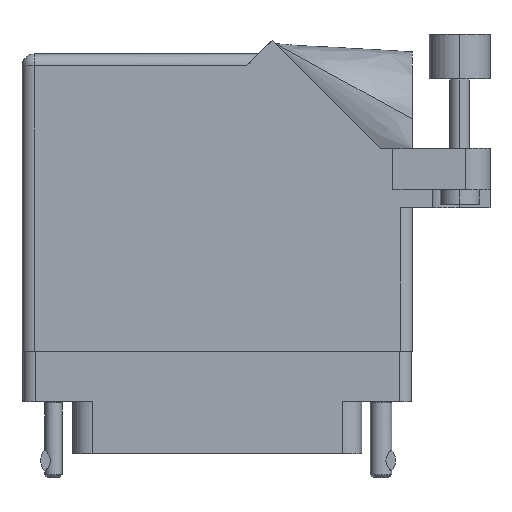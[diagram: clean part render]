
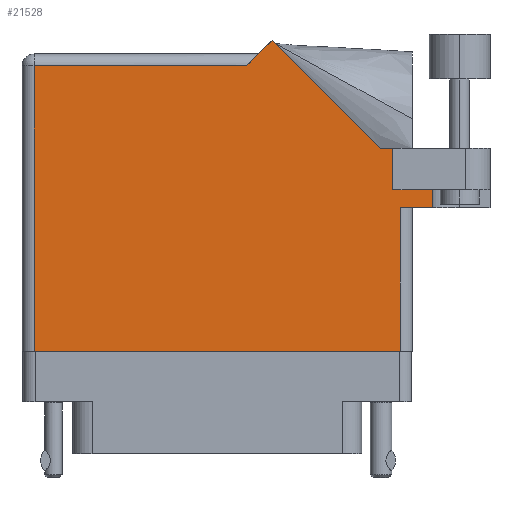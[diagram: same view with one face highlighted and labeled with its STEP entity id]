
A CAD part, front view. The second image highlights one B-rep face of the part: STEP entity #21528.
In plain terms, the highlighted face is planar.
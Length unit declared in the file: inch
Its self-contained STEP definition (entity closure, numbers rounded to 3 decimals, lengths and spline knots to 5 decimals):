
#61 = ORIENTED_EDGE ( 'NONE', *, *, #33246, .T. ) ;
#409 = ORIENTED_EDGE ( 'NONE', *, *, #46826, .F. ) ;
#610 = VERTEX_POINT ( 'NONE', #6853 ) ;
#816 = VERTEX_POINT ( 'NONE', #29741 ) ;
#1516 = DIRECTION ( 'NONE',  ( 0., 1., 0. ) ) ;
#3963 = CARTESIAN_POINT ( 'NONE',  ( 1.84442, 1.044, 0. ) ) ;
#4258 = VERTEX_POINT ( 'NONE', #4443 ) ;
#4443 = CARTESIAN_POINT ( 'NONE',  ( 0.062, 0., 0. ) ) ;
#5103 = DIRECTION ( 'NONE',  ( -0.707, 0.707, 0. ) ) ;
#5452 = ORIENTED_EDGE ( 'NONE', *, *, #24440, .T. ) ;
#6718 = CARTESIAN_POINT ( 'NONE',  ( 1.91, 0.831, 0. ) ) ;
#6816 = CARTESIAN_POINT ( 'NONE',  ( 1.91, 1.044, 0. ) ) ;
#6853 = CARTESIAN_POINT ( 'NONE',  ( 2.1115, 0.831, 0. ) ) ;
#7058 = VERTEX_POINT ( 'NONE', #6816 ) ;
#7632 = CARTESIAN_POINT ( 'NONE',  ( 0., 0., 0. ) ) ;
#8028 = ORIENTED_EDGE ( 'NONE', *, *, #10808, .T. ) ;
#9921 = DIRECTION ( 'NONE',  ( 0., -1., 0. ) ) ;
#10327 = VERTEX_POINT ( 'NONE', #3963 ) ;
#10651 = VECTOR ( 'NONE', #18929, 39.37008 ) ;
#10808 = EDGE_CURVE ( 'NONE', #44671, #12719, #25239, .T. ) ;
#11170 = CARTESIAN_POINT ( 'NONE',  ( 2.1115, 0.737, 0. ) ) ;
#11252 = PLANE ( 'NONE',  #29111 ) ;
#12719 = VERTEX_POINT ( 'NONE', #14755 ) ;
#13970 = CARTESIAN_POINT ( 'NONE',  ( 1.28771, 1.60071, 0. ) ) ;
#14287 = ORIENTED_EDGE ( 'NONE', *, *, #27732, .T. ) ;
#14678 = DIRECTION ( 'NONE',  ( 0., 0., -1. ) ) ;
#14755 = CARTESIAN_POINT ( 'NONE',  ( 1.948, 0.737, 0. ) ) ;
#16064 = DIRECTION ( 'NONE',  ( 1., 0., 0. ) ) ;
#16379 = DIRECTION ( 'NONE',  ( -0.707, -0.707, 0. ) ) ;
#16414 = LINE ( 'NONE', #7632, #10651 ) ;
#18099 = LINE ( 'NONE', #39887, #40368 ) ;
#18368 = CARTESIAN_POINT ( 'NONE',  ( 1.948, 0.737, 0. ) ) ;
#18465 = VERTEX_POINT ( 'NONE', #43264 ) ;
#18929 = DIRECTION ( 'NONE',  ( 1., 0., 0. ) ) ;
#19788 = ORIENTED_EDGE ( 'NONE', *, *, #43448, .T. ) ;
#19998 = CARTESIAN_POINT ( 'NONE',  ( 1.91, 0.831, 0. ) ) ;
#20545 = VECTOR ( 'NONE', #27353, 39.37008 ) ;
#20942 = VECTOR ( 'NONE', #5103, 39.37008 ) ;
#21034 = CARTESIAN_POINT ( 'NONE',  ( 1.948, 0., 0. ) ) ;
#21461 = VECTOR ( 'NONE', #16379, 39.37008 ) ;
#21528 = ADVANCED_FACE ( 'NONE', ( #33737 ), #11252, .F. ) ;
#21626 = DIRECTION ( 'NONE',  ( -1., 0., 0. ) ) ;
#21984 = LINE ( 'NONE', #31185, #29567 ) ;
#22434 = VECTOR ( 'NONE', #1516, 39.37008 ) ;
#22444 = LINE ( 'NONE', #32644, #28306 ) ;
#23491 = LINE ( 'NONE', #36527, #29917 ) ;
#24135 = LINE ( 'NONE', #46702, #29380 ) ;
#24164 = VERTEX_POINT ( 'NONE', #13970 ) ;
#24440 = EDGE_CURVE ( 'NONE', #44166, #7058, #44708, .T. ) ;
#25079 = ORIENTED_EDGE ( 'NONE', *, *, #25522, .T. ) ;
#25239 = LINE ( 'NONE', #18368, #37554 ) ;
#25510 = ORIENTED_EDGE ( 'NONE', *, *, #35827, .T. ) ;
#25522 = EDGE_CURVE ( 'NONE', #4258, #44671, #16414, .T. ) ;
#25665 = CARTESIAN_POINT ( 'NONE',  ( 0., 1.53, 0. ) ) ;
#27353 = DIRECTION ( 'NONE',  ( -1., 0., 0. ) ) ;
#27732 = EDGE_CURVE ( 'NONE', #12719, #35577, #18099, .T. ) ;
#27891 = DIRECTION ( 'NONE',  ( 0., -1., 0. ) ) ;
#28306 = VECTOR ( 'NONE', #9921, 39.37008 ) ;
#29111 = AXIS2_PLACEMENT_3D ( 'NONE', #25665, #14678, #44984 ) ;
#29380 = VECTOR ( 'NONE', #27891, 39.37008 ) ;
#29567 = VECTOR ( 'NONE', #16064, 39.37008 ) ;
#29741 = CARTESIAN_POINT ( 'NONE',  ( 0.062, 1.468, 0. ) ) ;
#29917 = VECTOR ( 'NONE', #21626, 39.37008 ) ;
#30909 = CARTESIAN_POINT ( 'NONE',  ( 1.84442, 1.044, 0. ) ) ;
#31185 = CARTESIAN_POINT ( 'NONE',  ( 1.91, 0.831, 0. ) ) ;
#31380 = LINE ( 'NONE', #46689, #21461 ) ;
#32325 = EDGE_CURVE ( 'NONE', #816, #4258, #22444, .T. ) ;
#32644 = CARTESIAN_POINT ( 'NONE',  ( 0.062, 0., 0. ) ) ;
#33014 = ORIENTED_EDGE ( 'NONE', *, *, #42207, .T. ) ;
#33246 = EDGE_CURVE ( 'NONE', #18465, #816, #23491, .T. ) ;
#33560 = ORIENTED_EDGE ( 'NONE', *, *, #44188, .F. ) ;
#33737 = FACE_OUTER_BOUND ( 'NONE', #41269, .T. ) ;
#35577 = VERTEX_POINT ( 'NONE', #11170 ) ;
#35827 = EDGE_CURVE ( 'NONE', #7058, #10327, #40478, .T. ) ;
#36527 = CARTESIAN_POINT ( 'NONE',  ( 0., 1.468, 0. ) ) ;
#37339 = LINE ( 'NONE', #30909, #20942 ) ;
#37554 = VECTOR ( 'NONE', #48150, 39.37008 ) ;
#38992 = CARTESIAN_POINT ( 'NONE',  ( 2.41, 1.044, 0. ) ) ;
#39887 = CARTESIAN_POINT ( 'NONE',  ( 2.01, 0.737, 0. ) ) ;
#40368 = VECTOR ( 'NONE', #43664, 39.37008 ) ;
#40478 = LINE ( 'NONE', #38992, #20545 ) ;
#41269 = EDGE_LOOP ( 'NONE', ( #25079, #8028, #14287, #409, #33560, #5452, #25510, #33014, #19788, #61, #44927 ) ) ;
#42207 = EDGE_CURVE ( 'NONE', #10327, #24164, #37339, .T. ) ;
#43264 = CARTESIAN_POINT ( 'NONE',  ( 1.155, 1.468, 0. ) ) ;
#43448 = EDGE_CURVE ( 'NONE', #24164, #18465, #31380, .T. ) ;
#43664 = DIRECTION ( 'NONE',  ( 1., 0., 0. ) ) ;
#44166 = VERTEX_POINT ( 'NONE', #6718 ) ;
#44188 = EDGE_CURVE ( 'NONE', #44166, #610, #21984, .T. ) ;
#44671 = VERTEX_POINT ( 'NONE', #21034 ) ;
#44708 = LINE ( 'NONE', #19998, #22434 ) ;
#44927 = ORIENTED_EDGE ( 'NONE', *, *, #32325, .T. ) ;
#44984 = DIRECTION ( 'NONE',  ( -1., 0., 0. ) ) ;
#46689 = CARTESIAN_POINT ( 'NONE',  ( 1.217, 1.53, 0. ) ) ;
#46702 = CARTESIAN_POINT ( 'NONE',  ( 2.1115, 1.16177, 0. ) ) ;
#46826 = EDGE_CURVE ( 'NONE', #610, #35577, #24135, .T. ) ;
#48150 = DIRECTION ( 'NONE',  ( 0., 1., 0. ) ) ;
